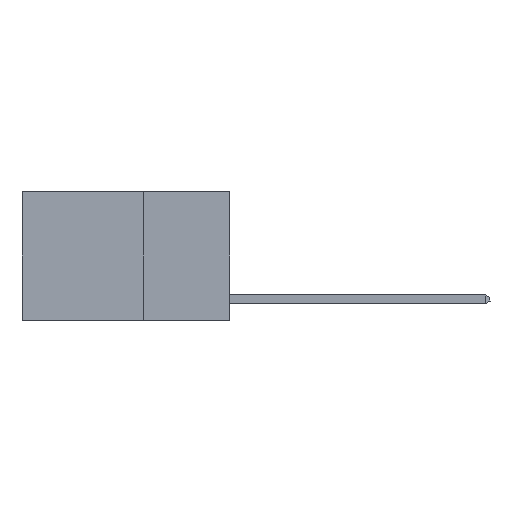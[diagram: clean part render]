
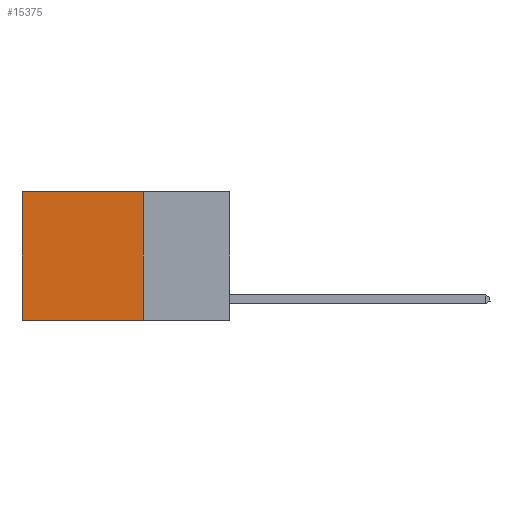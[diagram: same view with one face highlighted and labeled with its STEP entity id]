
A CAD part, left-side view. The second image highlights one B-rep face of the part: STEP entity #15375.
In plain terms, the highlighted planar face has unit normal (-1, 0, 0).
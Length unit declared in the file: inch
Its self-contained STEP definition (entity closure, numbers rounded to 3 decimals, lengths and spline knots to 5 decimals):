
#526 = VECTOR ( 'NONE', #10065, 39.37008 ) ;
#1786 = DIRECTION ( 'NONE',  ( 0., 1., 0. ) ) ;
#1944 = VERTEX_POINT ( 'NONE', #9407 ) ;
#2159 = VERTEX_POINT ( 'NONE', #2501 ) ;
#2501 = CARTESIAN_POINT ( 'NONE',  ( 0.2625, 0.25, -0.37 ) ) ;
#2681 = EDGE_CURVE ( 'NONE', #13605, #2159, #13176, .T. ) ;
#3051 = EDGE_CURVE ( 'NONE', #1944, #4079, #15687, .T. ) ;
#3355 = DIRECTION ( 'NONE',  ( 0., 0., -1. ) ) ;
#3849 = AXIS2_PLACEMENT_3D ( 'NONE', #13559, #7360, #9631 ) ;
#3977 = EDGE_CURVE ( 'NONE', #2159, #4079, #9392, .T. ) ;
#4079 = VERTEX_POINT ( 'NONE', #11877 ) ;
#5653 = LINE ( 'NONE', #14520, #11541 ) ;
#6041 = PLANE ( 'NONE',  #3849 ) ;
#6333 = ORIENTED_EDGE ( 'NONE', *, *, #2681, .F. ) ;
#6821 = VECTOR ( 'NONE', #1786, 39.37008 ) ;
#7360 = DIRECTION ( 'NONE',  ( 1., 0., 0. ) ) ;
#7621 = ORIENTED_EDGE ( 'NONE', *, *, #3977, .F. ) ;
#7710 = ORIENTED_EDGE ( 'NONE', *, *, #10113, .T. ) ;
#9392 = LINE ( 'NONE', #10821, #6821 ) ;
#9407 = CARTESIAN_POINT ( 'NONE',  ( 0.2625, 0.6, 0. ) ) ;
#9631 = DIRECTION ( 'NONE',  ( 0., 0., -1. ) ) ;
#10065 = DIRECTION ( 'NONE',  ( 0., 0., -1. ) ) ;
#10113 = EDGE_CURVE ( 'NONE', #13605, #1944, #5653, .T. ) ;
#10821 = CARTESIAN_POINT ( 'NONE',  ( 0.2625, 0.25, -0.37 ) ) ;
#11288 = ORIENTED_EDGE ( 'NONE', *, *, #3051, .T. ) ;
#11541 = VECTOR ( 'NONE', #15853, 39.37008 ) ;
#11877 = CARTESIAN_POINT ( 'NONE',  ( 0.2625, 0.6, -0.37 ) ) ;
#12310 = CARTESIAN_POINT ( 'NONE',  ( 0.2625, 0.6, 0. ) ) ;
#12497 = CARTESIAN_POINT ( 'NONE',  ( 0.2625, 0.25, 0. ) ) ;
#13176 = LINE ( 'NONE', #12497, #526 ) ;
#13559 = CARTESIAN_POINT ( 'NONE',  ( 0.2625, 0.25, 0. ) ) ;
#13605 = VERTEX_POINT ( 'NONE', #15447 ) ;
#14520 = CARTESIAN_POINT ( 'NONE',  ( 0.2625, 0.25, 0. ) ) ;
#14930 = FACE_OUTER_BOUND ( 'NONE', #15188, .T. ) ;
#15188 = EDGE_LOOP ( 'NONE', ( #11288, #7621, #6333, #7710 ) ) ;
#15300 = VECTOR ( 'NONE', #3355, 39.37008 ) ;
#15375 = ADVANCED_FACE ( 'NONE', ( #14930 ), #6041, .F. ) ;
#15447 = CARTESIAN_POINT ( 'NONE',  ( 0.2625, 0.25, 0. ) ) ;
#15687 = LINE ( 'NONE', #12310, #15300 ) ;
#15853 = DIRECTION ( 'NONE',  ( 0., 1., 0. ) ) ;
